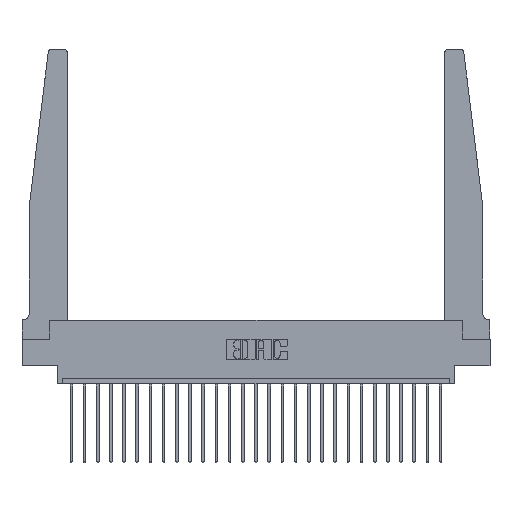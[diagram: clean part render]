
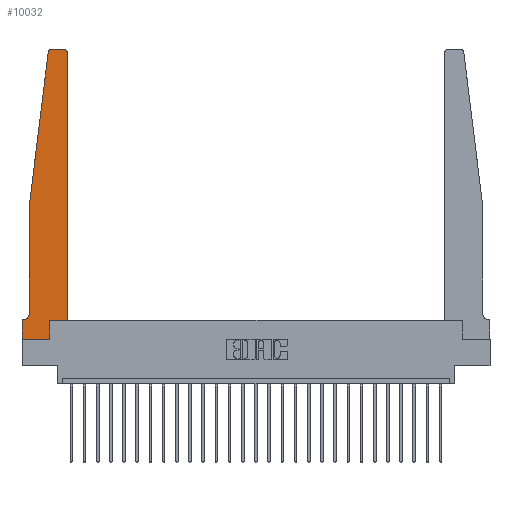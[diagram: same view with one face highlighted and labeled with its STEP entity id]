
A CAD part, top view. The second image highlights one B-rep face of the part: STEP entity #10032.
In plain terms, the highlighted planar face has unit normal (0, 0, 1).
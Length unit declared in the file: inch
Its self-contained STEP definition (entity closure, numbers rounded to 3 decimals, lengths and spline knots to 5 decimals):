
#421 = EDGE_CURVE ( 'NONE', #3433, #8180, #12277, .T. ) ;
#492 = VERTEX_POINT ( 'NONE', #3247 ) ;
#860 = VERTEX_POINT ( 'NONE', #21081 ) ;
#1020 = LINE ( 'NONE', #3870, #18646 ) ;
#1061 = CARTESIAN_POINT ( 'NONE',  ( 0.065, 1.25, 0.37 ) ) ;
#1172 = EDGE_CURVE ( 'NONE', #13240, #7366, #8105, .T. ) ;
#1338 = DIRECTION ( 'NONE',  ( 0., -1., 0. ) ) ;
#1482 = ORIENTED_EDGE ( 'NONE', *, *, #9686, .T. ) ;
#1616 = DIRECTION ( 'NONE',  ( -1., 0., 0. ) ) ;
#2067 = ORIENTED_EDGE ( 'NONE', *, *, #10552, .T. ) ;
#2308 = EDGE_LOOP ( 'NONE', ( #1482, #2067, #3929, #13749, #5087, #12883, #10092, #16328, #14497, #24621, #16918, #14312 ) ) ;
#2347 = DIRECTION ( 'NONE',  ( 0., 1., 0. ) ) ;
#2496 = CARTESIAN_POINT ( 'NONE',  ( 0.27653, 2.75, 0.37 ) ) ;
#2527 = LINE ( 'NONE', #22696, #12135 ) ;
#2711 = CIRCLE ( 'NONE', #11423, 0.03 ) ;
#2768 = PLANE ( 'NONE',  #10582 ) ;
#3247 = CARTESIAN_POINT ( 'NONE',  ( 0.425, 0.18, 0.37 ) ) ;
#3433 = VERTEX_POINT ( 'NONE', #1061 ) ;
#3786 = CIRCLE ( 'NONE', #11533, 0.03 ) ;
#3870 = CARTESIAN_POINT ( 'NONE',  ( 0.425, 0.18, 0.37 ) ) ;
#3929 = ORIENTED_EDGE ( 'NONE', *, *, #15544, .T. ) ;
#4390 = DIRECTION ( 'NONE',  ( 0., 0., 1. ) ) ;
#5075 = CARTESIAN_POINT ( 'NONE',  ( 0., 0., 0.37 ) ) ;
#5087 = ORIENTED_EDGE ( 'NONE', *, *, #7444, .T. ) ;
#5211 = DIRECTION ( 'NONE',  ( -1., 0., 0. ) ) ;
#5772 = VECTOR ( 'NONE', #8893, 39.37008 ) ;
#5860 = LINE ( 'NONE', #24485, #19869 ) ;
#5924 = CIRCLE ( 'NONE', #13255, 0.05 ) ;
#6730 = CARTESIAN_POINT ( 'NONE',  ( 0.015, 0.2375, 0.37 ) ) ;
#6993 = LINE ( 'NONE', #13090, #13559 ) ;
#7000 = DIRECTION ( 'NONE',  ( 1., 0., 0. ) ) ;
#7366 = VERTEX_POINT ( 'NONE', #20054 ) ;
#7444 = EDGE_CURVE ( 'NONE', #8180, #23627, #5924, .T. ) ;
#7552 = DIRECTION ( 'NONE',  ( 1., 0., 0. ) ) ;
#8105 = LINE ( 'NONE', #11378, #21524 ) ;
#8180 = VERTEX_POINT ( 'NONE', #22839 ) ;
#8385 = VECTOR ( 'NONE', #7000, 39.37008 ) ;
#8538 = CARTESIAN_POINT ( 'NONE',  ( 0., 0.1875, 0.37 ) ) ;
#8755 = VERTEX_POINT ( 'NONE', #22504 ) ;
#8893 = DIRECTION ( 'NONE',  ( -1., 0., 0. ) ) ;
#8925 = CARTESIAN_POINT ( 'NONE',  ( 0., 0.1875, 0.37 ) ) ;
#9164 = VERTEX_POINT ( 'NONE', #2496 ) ;
#9338 = VERTEX_POINT ( 'NONE', #20711 ) ;
#9660 = DIRECTION ( 'NONE',  ( 0., 0., 1. ) ) ;
#9686 = EDGE_CURVE ( 'NONE', #19070, #9164, #2527, .T. ) ;
#9772 = DIRECTION ( 'NONE',  ( -0.122, -0.992, 0. ) ) ;
#10032 = ADVANCED_FACE ( 'NONE', ( #11509 ), #2768, .T. ) ;
#10092 = ORIENTED_EDGE ( 'NONE', *, *, #1172, .T. ) ;
#10293 = CARTESIAN_POINT ( 'NONE',  ( 0.395, 2.75, 0.37 ) ) ;
#10552 = EDGE_CURVE ( 'NONE', #9164, #9338, #3786, .T. ) ;
#10582 = AXIS2_PLACEMENT_3D ( 'NONE', #8538, #12361, #22148 ) ;
#10850 = DIRECTION ( 'NONE',  ( 0., 0., -1. ) ) ;
#11105 = VECTOR ( 'NONE', #9772, 39.37008 ) ;
#11378 = CARTESIAN_POINT ( 'NONE',  ( 0., 0., 0.37 ) ) ;
#11423 = AXIS2_PLACEMENT_3D ( 'NONE', #22884, #9660, #22973 ) ;
#11509 = FACE_OUTER_BOUND ( 'NONE', #2308, .T. ) ;
#11533 = AXIS2_PLACEMENT_3D ( 'NONE', #23239, #4390, #17777 ) ;
#11697 = CARTESIAN_POINT ( 'NONE',  ( 0.015, 0.1875, 0.37 ) ) ;
#12135 = VECTOR ( 'NONE', #1616, 39.37008 ) ;
#12180 = CARTESIAN_POINT ( 'NONE',  ( 0.2605, 0.18, 0.37 ) ) ;
#12277 = LINE ( 'NONE', #19902, #19713 ) ;
#12361 = DIRECTION ( 'NONE',  ( 0., 0., 1. ) ) ;
#12883 = ORIENTED_EDGE ( 'NONE', *, *, #20021, .T. ) ;
#13090 = CARTESIAN_POINT ( 'NONE',  ( 0.425, 0.18, 0.37 ) ) ;
#13188 = LINE ( 'NONE', #15630, #11105 ) ;
#13240 = VERTEX_POINT ( 'NONE', #8925 ) ;
#13255 = AXIS2_PLACEMENT_3D ( 'NONE', #6730, #10850, #5211 ) ;
#13302 = DIRECTION ( 'NONE',  ( 0., -1., 0. ) ) ;
#13559 = VECTOR ( 'NONE', #16927, 39.37008 ) ;
#13749 = ORIENTED_EDGE ( 'NONE', *, *, #421, .T. ) ;
#14312 = ORIENTED_EDGE ( 'NONE', *, *, #14572, .T. ) ;
#14497 = ORIENTED_EDGE ( 'NONE', *, *, #20719, .T. ) ;
#14572 = EDGE_CURVE ( 'NONE', #8755, #19070, #2711, .T. ) ;
#14573 = CARTESIAN_POINT ( 'NONE',  ( 0.065, 0.1875, 0.37 ) ) ;
#14707 = LINE ( 'NONE', #5075, #8385 ) ;
#15544 = EDGE_CURVE ( 'NONE', #9338, #3433, #13188, .T. ) ;
#15630 = CARTESIAN_POINT ( 'NONE',  ( 0.065, 1.25, 0.37 ) ) ;
#15958 = VERTEX_POINT ( 'NONE', #12180 ) ;
#16328 = ORIENTED_EDGE ( 'NONE', *, *, #23243, .T. ) ;
#16918 = ORIENTED_EDGE ( 'NONE', *, *, #22182, .T. ) ;
#16927 = DIRECTION ( 'NONE',  ( 0., 1., 0. ) ) ;
#17777 = DIRECTION ( 'NONE',  ( 1., 0., 0. ) ) ;
#18646 = VECTOR ( 'NONE', #7552, 39.37008 ) ;
#19070 = VERTEX_POINT ( 'NONE', #10293 ) ;
#19713 = VECTOR ( 'NONE', #1338, 39.37008 ) ;
#19869 = VECTOR ( 'NONE', #2347, 39.37008 ) ;
#19902 = CARTESIAN_POINT ( 'NONE',  ( 0.065, 1.25, 0.37 ) ) ;
#20021 = EDGE_CURVE ( 'NONE', #23627, #13240, #21589, .T. ) ;
#20054 = CARTESIAN_POINT ( 'NONE',  ( 0., 0., 0.37 ) ) ;
#20711 = CARTESIAN_POINT ( 'NONE',  ( 0.24675, 2.72367, 0.37 ) ) ;
#20719 = EDGE_CURVE ( 'NONE', #860, #15958, #5860, .T. ) ;
#21081 = CARTESIAN_POINT ( 'NONE',  ( 0.2605, 0., 0.37 ) ) ;
#21524 = VECTOR ( 'NONE', #13302, 39.37008 ) ;
#21589 = LINE ( 'NONE', #14573, #5772 ) ;
#21593 = EDGE_CURVE ( 'NONE', #15958, #492, #1020, .T. ) ;
#22148 = DIRECTION ( 'NONE',  ( 1., 0., 0. ) ) ;
#22182 = EDGE_CURVE ( 'NONE', #492, #8755, #6993, .T. ) ;
#22504 = CARTESIAN_POINT ( 'NONE',  ( 0.425, 2.72, 0.37 ) ) ;
#22696 = CARTESIAN_POINT ( 'NONE',  ( 0.25, 2.75, 0.37 ) ) ;
#22839 = CARTESIAN_POINT ( 'NONE',  ( 0.065, 0.2375, 0.37 ) ) ;
#22884 = CARTESIAN_POINT ( 'NONE',  ( 0.395, 2.72, 0.37 ) ) ;
#22973 = DIRECTION ( 'NONE',  ( 1., 0., 0. ) ) ;
#23239 = CARTESIAN_POINT ( 'NONE',  ( 0.27653, 2.72, 0.37 ) ) ;
#23243 = EDGE_CURVE ( 'NONE', #7366, #860, #14707, .T. ) ;
#23627 = VERTEX_POINT ( 'NONE', #11697 ) ;
#24485 = CARTESIAN_POINT ( 'NONE',  ( 0.2605, 0.18, 0.37 ) ) ;
#24621 = ORIENTED_EDGE ( 'NONE', *, *, #21593, .T. ) ;
